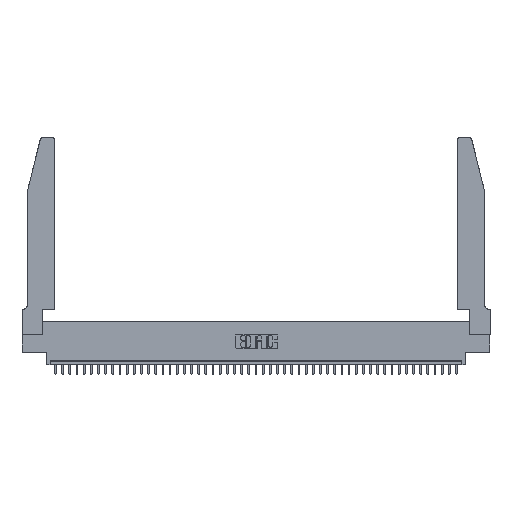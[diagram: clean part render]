
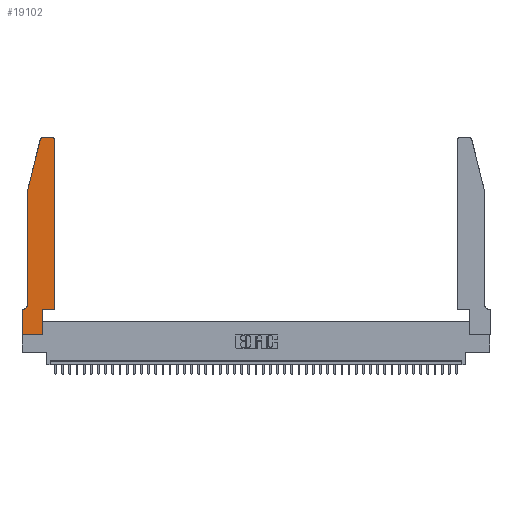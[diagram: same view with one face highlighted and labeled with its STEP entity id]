
A CAD part, top view. The second image highlights one B-rep face of the part: STEP entity #19102.
In plain terms, the highlighted planar face has unit normal (0, 0, 1).
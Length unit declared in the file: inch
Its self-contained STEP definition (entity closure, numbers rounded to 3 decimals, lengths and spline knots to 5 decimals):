
#257 = VECTOR ( 'NONE', #41351, 39.37008 ) ;
#1331 = LINE ( 'NONE', #17812, #35661 ) ;
#2004 = AXIS2_PLACEMENT_3D ( 'NONE', #4751, #8495, #7869 ) ;
#2498 = VECTOR ( 'NONE', #33278, 39.37008 ) ;
#2651 = ORIENTED_EDGE ( 'NONE', *, *, #27358, .T. ) ;
#2735 = DIRECTION ( 'NONE',  ( 0., -1., 0. ) ) ;
#2768 = EDGE_CURVE ( 'NONE', #6796, #21729, #39605, .T. ) ;
#3555 = AXIS2_PLACEMENT_3D ( 'NONE', #8212, #39713, #25481 ) ;
#4610 = CARTESIAN_POINT ( 'NONE',  ( 0.2865, 0.35, 0.37 ) ) ;
#4751 = CARTESIAN_POINT ( 'NONE',  ( 0.0055, 0.42, 0.37 ) ) ;
#5089 = CARTESIAN_POINT ( 'NONE',  ( 0.4205, 2.72, 0.37 ) ) ;
#5333 = CARTESIAN_POINT ( 'NONE',  ( 0.0755, 0.35, 0.37 ) ) ;
#6366 = LINE ( 'NONE', #39460, #7439 ) ;
#6796 = VERTEX_POINT ( 'NONE', #13176 ) ;
#7177 = EDGE_CURVE ( 'NONE', #21514, #26517, #8858, .T. ) ;
#7439 = VECTOR ( 'NONE', #15232, 39.37008 ) ;
#7869 = DIRECTION ( 'NONE',  ( -1., 0., 0. ) ) ;
#7889 = CIRCLE ( 'NONE', #3555, 0.03 ) ;
#8093 = CARTESIAN_POINT ( 'NONE',  ( 0.0755, 2., 0.37 ) ) ;
#8212 = CARTESIAN_POINT ( 'NONE',  ( 0.284, 2.72, 0.37 ) ) ;
#8495 = DIRECTION ( 'NONE',  ( 0., 0., -1. ) ) ;
#8858 = LINE ( 'NONE', #41299, #33729 ) ;
#9812 = EDGE_LOOP ( 'NONE', ( #32132, #17215, #43626, #33034, #41154, #2651, #16266, #20710, #21267, #31231, #28112, #13635 ) ) ;
#9855 = DIRECTION ( 'NONE',  ( 0., 0., 1. ) ) ;
#10009 = DIRECTION ( 'NONE',  ( -1., 0., 0. ) ) ;
#10566 = DIRECTION ( 'NONE',  ( -1., 0., 0. ) ) ;
#11630 = CARTESIAN_POINT ( 'NONE',  ( 0., 0., 0.37 ) ) ;
#13176 = CARTESIAN_POINT ( 'NONE',  ( 0.0755, 2., 0.37 ) ) ;
#13635 = ORIENTED_EDGE ( 'NONE', *, *, #39365, .T. ) ;
#15232 = DIRECTION ( 'NONE',  ( 1., 0., 0. ) ) ;
#16266 = ORIENTED_EDGE ( 'NONE', *, *, #30387, .T. ) ;
#16300 = EDGE_CURVE ( 'NONE', #21184, #27924, #25521, .T. ) ;
#16685 = VERTEX_POINT ( 'NONE', #11630 ) ;
#17215 = ORIENTED_EDGE ( 'NONE', *, *, #37501, .T. ) ;
#17812 = CARTESIAN_POINT ( 'NONE',  ( 0.2605, 2.75, 0.37 ) ) ;
#17971 = CIRCLE ( 'NONE', #2004, 0.07 ) ;
#19102 = ADVANCED_FACE ( 'NONE', ( #27482 ), #45374, .T. ) ;
#20337 = EDGE_CURVE ( 'NONE', #27924, #21514, #6366, .T. ) ;
#20495 = CARTESIAN_POINT ( 'NONE',  ( 0., 0., 0.37 ) ) ;
#20536 = CARTESIAN_POINT ( 'NONE',  ( 0.0755, 2., 0.37 ) ) ;
#20710 = ORIENTED_EDGE ( 'NONE', *, *, #44753, .T. ) ;
#21184 = VERTEX_POINT ( 'NONE', #41234 ) ;
#21267 = ORIENTED_EDGE ( 'NONE', *, *, #16300, .T. ) ;
#21514 = VERTEX_POINT ( 'NONE', #22570 ) ;
#21729 = VERTEX_POINT ( 'NONE', #21749 ) ;
#21749 = CARTESIAN_POINT ( 'NONE',  ( 0.0755, 0.42, 0.37 ) ) ;
#22570 = CARTESIAN_POINT ( 'NONE',  ( 0.4505, 0.35, 0.37 ) ) ;
#23054 = VECTOR ( 'NONE', #2735, 39.37008 ) ;
#23363 = VECTOR ( 'NONE', #35088, 39.37008 ) ;
#23770 = CARTESIAN_POINT ( 'NONE',  ( 0., 0., 0.37 ) ) ;
#24327 = CARTESIAN_POINT ( 'NONE',  ( 0.2865, 0.35, 0.37 ) ) ;
#25175 = AXIS2_PLACEMENT_3D ( 'NONE', #5089, #36777, #33719 ) ;
#25481 = DIRECTION ( 'NONE',  ( 1., 0., 0. ) ) ;
#25521 = LINE ( 'NONE', #4610, #23363 ) ;
#26517 = VERTEX_POINT ( 'NONE', #37481 ) ;
#26924 = VERTEX_POINT ( 'NONE', #43527 ) ;
#27358 = EDGE_CURVE ( 'NONE', #29008, #35578, #36820, .T. ) ;
#27482 = FACE_OUTER_BOUND ( 'NONE', #9812, .T. ) ;
#27725 = CARTESIAN_POINT ( 'NONE',  ( 0., 0.35, 0.37 ) ) ;
#27887 = CARTESIAN_POINT ( 'NONE',  ( 0., 0.35, 0.37 ) ) ;
#27924 = VERTEX_POINT ( 'NONE', #24327 ) ;
#28112 = ORIENTED_EDGE ( 'NONE', *, *, #7177, .T. ) ;
#28225 = EDGE_CURVE ( 'NONE', #45158, #6796, #29562, .T. ) ;
#28289 = CARTESIAN_POINT ( 'NONE',  ( 0.4205, 2.75, 0.37 ) ) ;
#28738 = EDGE_CURVE ( 'NONE', #21729, #29008, #17971, .T. ) ;
#29008 = VERTEX_POINT ( 'NONE', #33026 ) ;
#29562 = LINE ( 'NONE', #8093, #2498 ) ;
#30387 = EDGE_CURVE ( 'NONE', #35578, #16685, #36023, .T. ) ;
#31231 = ORIENTED_EDGE ( 'NONE', *, *, #20337, .T. ) ;
#31526 = CIRCLE ( 'NONE', #25175, 0.03 ) ;
#32132 = ORIENTED_EDGE ( 'NONE', *, *, #41724, .T. ) ;
#32944 = CARTESIAN_POINT ( 'NONE',  ( 0.25487, 2.72718, 0.37 ) ) ;
#33026 = CARTESIAN_POINT ( 'NONE',  ( 0.0055, 0.35, 0.37 ) ) ;
#33034 = ORIENTED_EDGE ( 'NONE', *, *, #2768, .T. ) ;
#33278 = DIRECTION ( 'NONE',  ( -0.239, -0.971, 0. ) ) ;
#33719 = DIRECTION ( 'NONE',  ( 1., 0., 0. ) ) ;
#33729 = VECTOR ( 'NONE', #38523, 39.37008 ) ;
#34566 = DIRECTION ( 'NONE',  ( 1., 0., 0. ) ) ;
#35088 = DIRECTION ( 'NONE',  ( 0., 1., 0. ) ) ;
#35578 = VERTEX_POINT ( 'NONE', #27887 ) ;
#35618 = LINE ( 'NONE', #20495, #257 ) ;
#35661 = VECTOR ( 'NONE', #10566, 39.37008 ) ;
#35730 = VECTOR ( 'NONE', #10009, 39.37008 ) ;
#36023 = LINE ( 'NONE', #23770, #42152 ) ;
#36777 = DIRECTION ( 'NONE',  ( 0., 0., 1. ) ) ;
#36820 = LINE ( 'NONE', #5333, #35730 ) ;
#36858 = VERTEX_POINT ( 'NONE', #28289 ) ;
#37481 = CARTESIAN_POINT ( 'NONE',  ( 0.4505, 2.72, 0.37 ) ) ;
#37501 = EDGE_CURVE ( 'NONE', #26924, #45158, #7889, .T. ) ;
#38523 = DIRECTION ( 'NONE',  ( 0., 1., 0. ) ) ;
#39365 = EDGE_CURVE ( 'NONE', #26517, #36858, #31526, .T. ) ;
#39460 = CARTESIAN_POINT ( 'NONE',  ( 0.4505, 0.35, 0.37 ) ) ;
#39605 = LINE ( 'NONE', #20536, #23054 ) ;
#39713 = DIRECTION ( 'NONE',  ( 0., 0., 1. ) ) ;
#41154 = ORIENTED_EDGE ( 'NONE', *, *, #28738, .T. ) ;
#41234 = CARTESIAN_POINT ( 'NONE',  ( 0.2865, 0., 0.37 ) ) ;
#41299 = CARTESIAN_POINT ( 'NONE',  ( 0.4505, 0.35, 0.37 ) ) ;
#41351 = DIRECTION ( 'NONE',  ( 1., 0., 0. ) ) ;
#41724 = EDGE_CURVE ( 'NONE', #36858, #26924, #1331, .T. ) ;
#42152 = VECTOR ( 'NONE', #45097, 39.37008 ) ;
#42397 = AXIS2_PLACEMENT_3D ( 'NONE', #27725, #9855, #34566 ) ;
#43527 = CARTESIAN_POINT ( 'NONE',  ( 0.284, 2.75, 0.37 ) ) ;
#43626 = ORIENTED_EDGE ( 'NONE', *, *, #28225, .T. ) ;
#44753 = EDGE_CURVE ( 'NONE', #16685, #21184, #35618, .T. ) ;
#45097 = DIRECTION ( 'NONE',  ( 0., -1., 0. ) ) ;
#45158 = VERTEX_POINT ( 'NONE', #32944 ) ;
#45374 = PLANE ( 'NONE',  #42397 ) ;
